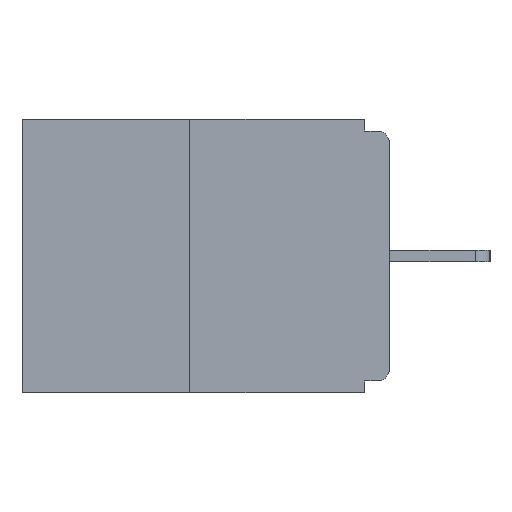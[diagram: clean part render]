
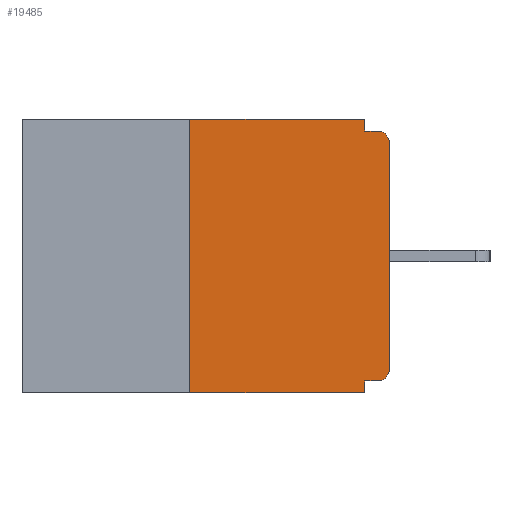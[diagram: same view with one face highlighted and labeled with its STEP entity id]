
A CAD part, left-side view. The second image highlights one B-rep face of the part: STEP entity #19485.
In plain terms, the highlighted planar face has unit normal (-1, 0, 0).
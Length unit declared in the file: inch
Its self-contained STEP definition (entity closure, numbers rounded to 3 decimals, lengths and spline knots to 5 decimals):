
#179 = LINE ( 'NONE', #23381, #5261 ) ;
#789 = VECTOR ( 'NONE', #11381, 39.37008 ) ;
#894 = CIRCLE ( 'NONE', #19930, 0.015 ) ;
#989 = CARTESIAN_POINT ( 'NONE',  ( 0., 0.031, -0.328 ) ) ;
#1342 = VECTOR ( 'NONE', #8463, 39.37008 ) ;
#2066 = DIRECTION ( 'NONE',  ( 1., 0., 0. ) ) ;
#2335 = CARTESIAN_POINT ( 'NONE',  ( 0., 0.031, -0.343 ) ) ;
#2754 = LINE ( 'NONE', #18082, #1342 ) ;
#3059 = ORIENTED_EDGE ( 'NONE', *, *, #12630, .T. ) ;
#3077 = EDGE_CURVE ( 'NONE', #23186, #5880, #2754, .T. ) ;
#3117 = ORIENTED_EDGE ( 'NONE', *, *, #23788, .T. ) ;
#3596 = LINE ( 'NONE', #19065, #19024 ) ;
#3869 = CARTESIAN_POINT ( 'NONE',  ( 0., 0.46, -0.343 ) ) ;
#4585 = ORIENTED_EDGE ( 'NONE', *, *, #22062, .F. ) ;
#5013 = EDGE_CURVE ( 'NONE', #8191, #17444, #11746, .T. ) ;
#5195 = CARTESIAN_POINT ( 'NONE',  ( 0., 0.015, -0.328 ) ) ;
#5261 = VECTOR ( 'NONE', #25023, 39.37008 ) ;
#5843 = EDGE_LOOP ( 'NONE', ( #12585, #4585, #3117, #19842, #22925, #3059, #9136, #19498, #20306, #16213 ) ) ;
#5873 = DIRECTION ( 'NONE',  ( 0., 1., 0. ) ) ;
#5880 = VERTEX_POINT ( 'NONE', #11982 ) ;
#7267 = DIRECTION ( 'NONE',  ( 0., 0., -1. ) ) ;
#7315 = VERTEX_POINT ( 'NONE', #14267 ) ;
#8191 = VERTEX_POINT ( 'NONE', #989 ) ;
#8463 = DIRECTION ( 'NONE',  ( 0., -1., 0. ) ) ;
#8503 = VERTEX_POINT ( 'NONE', #19851 ) ;
#9049 = DIRECTION ( 'NONE',  ( -1., 0., 0. ) ) ;
#9136 = ORIENTED_EDGE ( 'NONE', *, *, #17333, .T. ) ;
#9176 = LINE ( 'NONE', #11200, #10385 ) ;
#9309 = DIRECTION ( 'NONE',  ( 0., 0., 1. ) ) ;
#9589 = LINE ( 'NONE', #17201, #22595 ) ;
#10202 = DIRECTION ( 'NONE',  ( 0., 0., -1. ) ) ;
#10385 = VECTOR ( 'NONE', #9309, 39.37008 ) ;
#10655 = CARTESIAN_POINT ( 'NONE',  ( 0., 0.46, 0. ) ) ;
#11069 = DIRECTION ( 'NONE',  ( -1., 0., 0. ) ) ;
#11200 = CARTESIAN_POINT ( 'NONE',  ( 0., 0., 0. ) ) ;
#11288 = EDGE_CURVE ( 'NONE', #8503, #5880, #21081, .T. ) ;
#11331 = CARTESIAN_POINT ( 'NONE',  ( 0., 0.25, 0. ) ) ;
#11381 = DIRECTION ( 'NONE',  ( 0., -1., 0. ) ) ;
#11746 = LINE ( 'NONE', #2335, #18548 ) ;
#11982 = CARTESIAN_POINT ( 'NONE',  ( 0., 0.015, -0.015 ) ) ;
#12001 = VERTEX_POINT ( 'NONE', #14075 ) ;
#12087 = CARTESIAN_POINT ( 'NONE',  ( 0., 0.46, 0. ) ) ;
#12585 = ORIENTED_EDGE ( 'NONE', *, *, #14100, .F. ) ;
#12630 = EDGE_CURVE ( 'NONE', #24906, #22122, #894, .T. ) ;
#13125 = CARTESIAN_POINT ( 'NONE',  ( 0., 0.015, -0.03 ) ) ;
#13443 = AXIS2_PLACEMENT_3D ( 'NONE', #13125, #9049, #7267 ) ;
#14075 = CARTESIAN_POINT ( 'NONE',  ( 0., 0.25, -0.343 ) ) ;
#14100 = EDGE_CURVE ( 'NONE', #16735, #7315, #20143, .T. ) ;
#14267 = CARTESIAN_POINT ( 'NONE',  ( 0., 0.031, 0. ) ) ;
#14631 = CARTESIAN_POINT ( 'NONE',  ( 0., 0.031, -0.015 ) ) ;
#14927 = AXIS2_PLACEMENT_3D ( 'NONE', #12087, #2066, #21561 ) ;
#16213 = ORIENTED_EDGE ( 'NONE', *, *, #23760, .F. ) ;
#16735 = VERTEX_POINT ( 'NONE', #11331 ) ;
#17201 = CARTESIAN_POINT ( 'NONE',  ( 0., 0.25, 0. ) ) ;
#17320 = DIRECTION ( 'NONE',  ( 0., 0., 1. ) ) ;
#17333 = EDGE_CURVE ( 'NONE', #22122, #8503, #9176, .T. ) ;
#17444 = VERTEX_POINT ( 'NONE', #23456 ) ;
#17537 = FACE_OUTER_BOUND ( 'NONE', #5843, .T. ) ;
#18082 = CARTESIAN_POINT ( 'NONE',  ( 0., 0., -0.015 ) ) ;
#18548 = VECTOR ( 'NONE', #10202, 39.37008 ) ;
#19024 = VECTOR ( 'NONE', #5873, 39.37008 ) ;
#19065 = CARTESIAN_POINT ( 'NONE',  ( 0., 0., -0.328 ) ) ;
#19485 = ADVANCED_FACE ( 'NONE', ( #17537 ), #23457, .F. ) ;
#19498 = ORIENTED_EDGE ( 'NONE', *, *, #11288, .T. ) ;
#19842 = ORIENTED_EDGE ( 'NONE', *, *, #5013, .F. ) ;
#19851 = CARTESIAN_POINT ( 'NONE',  ( 0., 0., -0.03 ) ) ;
#19930 = AXIS2_PLACEMENT_3D ( 'NONE', #20808, #11069, #22957 ) ;
#20143 = LINE ( 'NONE', #10655, #22395 ) ;
#20306 = ORIENTED_EDGE ( 'NONE', *, *, #3077, .F. ) ;
#20808 = CARTESIAN_POINT ( 'NONE',  ( 0., 0.015, -0.313 ) ) ;
#21081 = CIRCLE ( 'NONE', #13443, 0.015 ) ;
#21229 = LINE ( 'NONE', #3869, #789 ) ;
#21561 = DIRECTION ( 'NONE',  ( 0., 0., -1. ) ) ;
#22062 = EDGE_CURVE ( 'NONE', #12001, #16735, #9589, .T. ) ;
#22122 = VERTEX_POINT ( 'NONE', #23248 ) ;
#22395 = VECTOR ( 'NONE', #24191, 39.37008 ) ;
#22595 = VECTOR ( 'NONE', #17320, 39.37008 ) ;
#22925 = ORIENTED_EDGE ( 'NONE', *, *, #24235, .F. ) ;
#22957 = DIRECTION ( 'NONE',  ( 0., 0., -1. ) ) ;
#23186 = VERTEX_POINT ( 'NONE', #14631 ) ;
#23248 = CARTESIAN_POINT ( 'NONE',  ( 0., 0., -0.313 ) ) ;
#23381 = CARTESIAN_POINT ( 'NONE',  ( 0., 0.031, 0. ) ) ;
#23456 = CARTESIAN_POINT ( 'NONE',  ( 0., 0.031, -0.343 ) ) ;
#23457 = PLANE ( 'NONE',  #14927 ) ;
#23760 = EDGE_CURVE ( 'NONE', #7315, #23186, #179, .T. ) ;
#23788 = EDGE_CURVE ( 'NONE', #12001, #17444, #21229, .T. ) ;
#24191 = DIRECTION ( 'NONE',  ( 0., -1., 0. ) ) ;
#24235 = EDGE_CURVE ( 'NONE', #24906, #8191, #3596, .T. ) ;
#24906 = VERTEX_POINT ( 'NONE', #5195 ) ;
#25023 = DIRECTION ( 'NONE',  ( 0., 0., -1. ) ) ;
